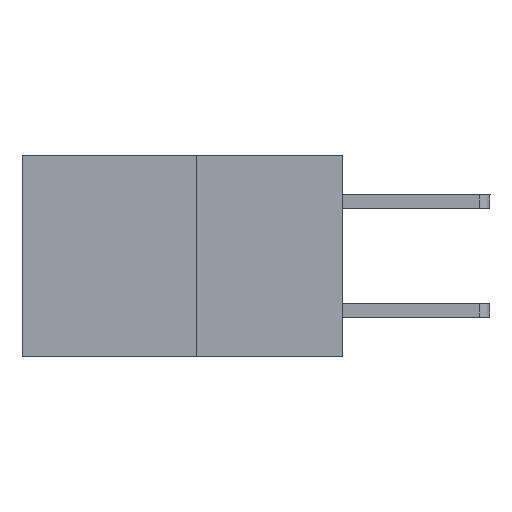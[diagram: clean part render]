
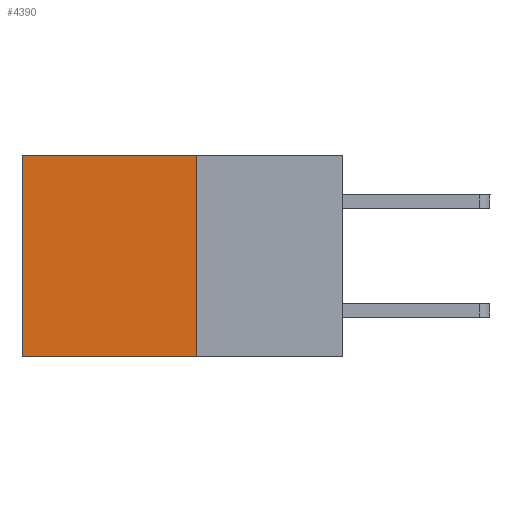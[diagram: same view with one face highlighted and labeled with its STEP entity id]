
A CAD part, left-side view. The second image highlights one B-rep face of the part: STEP entity #4390.
In plain terms, the highlighted planar face has unit normal (-1, 0, 0).
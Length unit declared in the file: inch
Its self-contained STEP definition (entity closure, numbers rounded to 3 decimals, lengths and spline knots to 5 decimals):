
#104 = DIRECTION ( 'NONE',  ( 1., 0., 0. ) ) ;
#686 = DIRECTION ( 'NONE',  ( 0., 1., 0. ) ) ;
#1360 = EDGE_CURVE ( 'NONE', #10817, #1905, #4841, .T. ) ;
#1372 = EDGE_CURVE ( 'NONE', #1905, #9277, #3262, .T. ) ;
#1524 = CARTESIAN_POINT ( 'NONE',  ( 0.277, 0.27, -0.37 ) ) ;
#1885 = CARTESIAN_POINT ( 'NONE',  ( 0.277, 0.27, -0.37 ) ) ;
#1905 = VERTEX_POINT ( 'NONE', #6831 ) ;
#2163 = VECTOR ( 'NONE', #10304, 39.37008 ) ;
#2422 = DIRECTION ( 'NONE',  ( 0., 0., -1. ) ) ;
#2935 = ORIENTED_EDGE ( 'NONE', *, *, #1360, .F. ) ;
#3262 = LINE ( 'NONE', #1524, #10657 ) ;
#3523 = DIRECTION ( 'NONE',  ( 0., 0., -1. ) ) ;
#3932 = VERTEX_POINT ( 'NONE', #8627 ) ;
#4060 = CARTESIAN_POINT ( 'NONE',  ( 0.277, 0.27, -0.37 ) ) ;
#4390 = ADVANCED_FACE ( 'NONE', ( #9558 ), #4534, .F. ) ;
#4501 = EDGE_LOOP ( 'NONE', ( #9884, #9714, #2935, #8864 ) ) ;
#4534 = PLANE ( 'NONE',  #6608 ) ;
#4841 = LINE ( 'NONE', #4060, #6349 ) ;
#6221 = EDGE_CURVE ( 'NONE', #3932, #9277, #9557, .T. ) ;
#6349 = VECTOR ( 'NONE', #2422, 39.37008 ) ;
#6608 = AXIS2_PLACEMENT_3D ( 'NONE', #1885, #104, #3523 ) ;
#6831 = CARTESIAN_POINT ( 'NONE',  ( 0.277, 0.27, -0.37 ) ) ;
#6878 = CARTESIAN_POINT ( 'NONE',  ( 0.277, 0.59, -0.37 ) ) ;
#7110 = VECTOR ( 'NONE', #10159, 39.37008 ) ;
#7199 = CARTESIAN_POINT ( 'NONE',  ( 0.277, 0.59, -0.37 ) ) ;
#7571 = CARTESIAN_POINT ( 'NONE',  ( 0.277, 0.27, 0. ) ) ;
#8627 = CARTESIAN_POINT ( 'NONE',  ( 0.277, 0.59, 0. ) ) ;
#8802 = CARTESIAN_POINT ( 'NONE',  ( 0.277, 0.27, 0. ) ) ;
#8864 = ORIENTED_EDGE ( 'NONE', *, *, #9739, .T. ) ;
#9140 = LINE ( 'NONE', #7571, #7110 ) ;
#9277 = VERTEX_POINT ( 'NONE', #7199 ) ;
#9557 = LINE ( 'NONE', #6878, #2163 ) ;
#9558 = FACE_OUTER_BOUND ( 'NONE', #4501, .T. ) ;
#9714 = ORIENTED_EDGE ( 'NONE', *, *, #1372, .F. ) ;
#9739 = EDGE_CURVE ( 'NONE', #10817, #3932, #9140, .T. ) ;
#9884 = ORIENTED_EDGE ( 'NONE', *, *, #6221, .T. ) ;
#10159 = DIRECTION ( 'NONE',  ( 0., 1., 0. ) ) ;
#10304 = DIRECTION ( 'NONE',  ( 0., 0., -1. ) ) ;
#10657 = VECTOR ( 'NONE', #686, 39.37008 ) ;
#10817 = VERTEX_POINT ( 'NONE', #8802 ) ;
